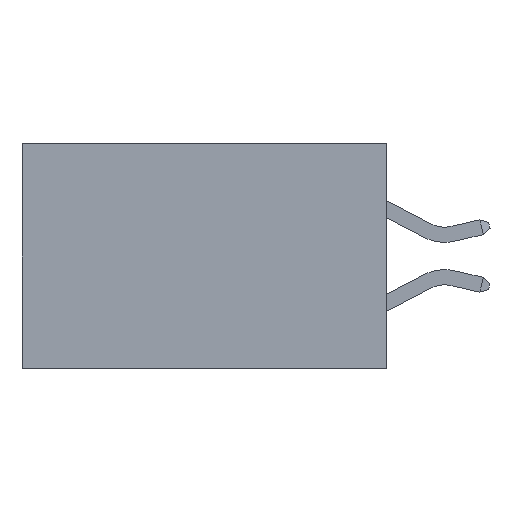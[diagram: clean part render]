
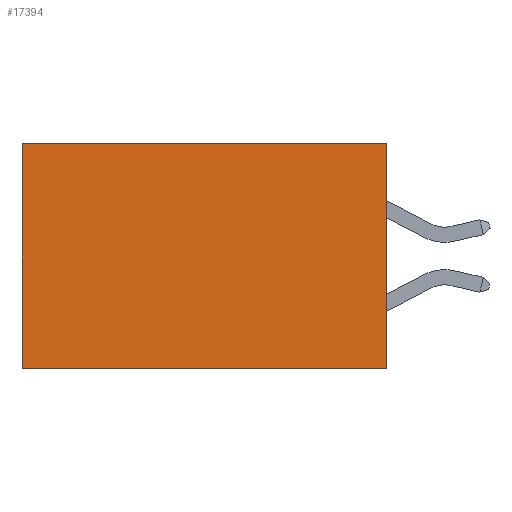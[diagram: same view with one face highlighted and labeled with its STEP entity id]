
A CAD part, left-side view. The second image highlights one B-rep face of the part: STEP entity #17394.
In plain terms, the highlighted planar face has unit normal (-1, 0, 0).
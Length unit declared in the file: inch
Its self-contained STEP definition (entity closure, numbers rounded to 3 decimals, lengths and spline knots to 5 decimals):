
#1751 = LINE ( 'NONE', #24256, #13282 ) ;
#2332 = PLANE ( 'NONE',  #11473 ) ;
#2458 = CARTESIAN_POINT ( 'NONE',  ( 0.2615, 0., -0.37 ) ) ;
#2635 = VERTEX_POINT ( 'NONE', #23322 ) ;
#3323 = VECTOR ( 'NONE', #21644, 39.37008 ) ;
#3331 = EDGE_CURVE ( 'NONE', #6292, #11676, #1751, .T. ) ;
#4029 = ORIENTED_EDGE ( 'NONE', *, *, #4344, .F. ) ;
#4344 = EDGE_CURVE ( 'NONE', #6312, #2635, #23986, .T. ) ;
#5081 = CARTESIAN_POINT ( 'NONE',  ( 0.2615, 0., -0.37 ) ) ;
#6292 = VERTEX_POINT ( 'NONE', #15004 ) ;
#6312 = VERTEX_POINT ( 'NONE', #22566 ) ;
#8468 = VECTOR ( 'NONE', #13719, 39.37008 ) ;
#9535 = VECTOR ( 'NONE', #10222, 39.37008 ) ;
#9894 = LINE ( 'NONE', #17305, #8468 ) ;
#10222 = DIRECTION ( 'NONE',  ( 0., 0., -1. ) ) ;
#11129 = CARTESIAN_POINT ( 'NONE',  ( 0.2615, 0.6, 0. ) ) ;
#11473 = AXIS2_PLACEMENT_3D ( 'NONE', #2458, #13805, #21371 ) ;
#11676 = VERTEX_POINT ( 'NONE', #11129 ) ;
#13212 = EDGE_CURVE ( 'NONE', #6292, #6312, #9894, .T. ) ;
#13282 = VECTOR ( 'NONE', #16842, 39.37008 ) ;
#13719 = DIRECTION ( 'NONE',  ( 0., 0., -1. ) ) ;
#13805 = DIRECTION ( 'NONE',  ( 1., 0., 0. ) ) ;
#15004 = CARTESIAN_POINT ( 'NONE',  ( 0.2615, 0., 0. ) ) ;
#16842 = DIRECTION ( 'NONE',  ( 0., 1., 0. ) ) ;
#17305 = CARTESIAN_POINT ( 'NONE',  ( 0.2615, 0., -0.37 ) ) ;
#17394 = ADVANCED_FACE ( 'NONE', ( #21117 ), #2332, .F. ) ;
#19753 = ORIENTED_EDGE ( 'NONE', *, *, #13212, .F. ) ;
#19873 = CARTESIAN_POINT ( 'NONE',  ( 0.2615, 0.6, -0.37 ) ) ;
#20456 = EDGE_CURVE ( 'NONE', #11676, #2635, #23336, .T. ) ;
#21117 = FACE_OUTER_BOUND ( 'NONE', #23184, .T. ) ;
#21371 = DIRECTION ( 'NONE',  ( 0., 0., -1. ) ) ;
#21425 = ORIENTED_EDGE ( 'NONE', *, *, #3331, .T. ) ;
#21644 = DIRECTION ( 'NONE',  ( 0., 1., 0. ) ) ;
#21712 = ORIENTED_EDGE ( 'NONE', *, *, #20456, .T. ) ;
#22566 = CARTESIAN_POINT ( 'NONE',  ( 0.2615, 0., -0.37 ) ) ;
#23184 = EDGE_LOOP ( 'NONE', ( #21712, #4029, #19753, #21425 ) ) ;
#23322 = CARTESIAN_POINT ( 'NONE',  ( 0.2615, 0.6, -0.37 ) ) ;
#23336 = LINE ( 'NONE', #19873, #9535 ) ;
#23986 = LINE ( 'NONE', #5081, #3323 ) ;
#24256 = CARTESIAN_POINT ( 'NONE',  ( 0.2615, 0., 0. ) ) ;
